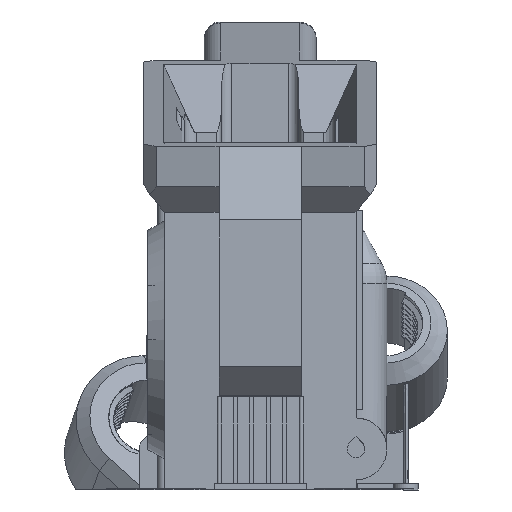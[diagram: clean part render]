
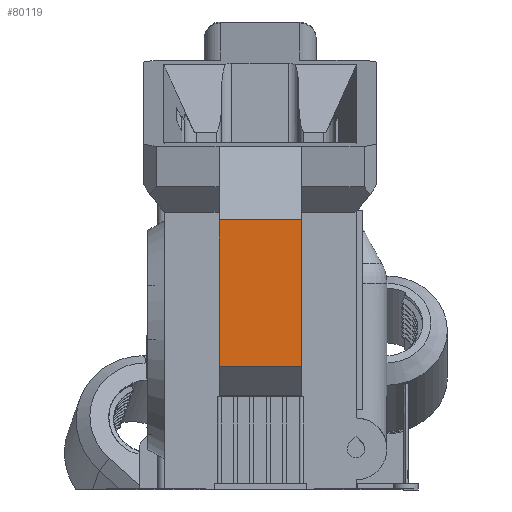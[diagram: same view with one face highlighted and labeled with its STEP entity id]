
A CAD part, left-side view. The second image highlights one B-rep face of the part: STEP entity #80119.
In plain terms, the highlighted planar face has unit normal (-1, 0, 0).
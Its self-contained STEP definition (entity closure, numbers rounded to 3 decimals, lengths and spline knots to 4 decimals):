
#517 = DIRECTION ( 'NONE',  ( 0., 0., 1. ) ) ;
#813 = EDGE_CURVE ( 'NONE', #81451, #173788, #107003, .T. ) ;
#8181 = VERTEX_POINT ( 'NONE', #47646 ) ;
#12141 = LINE ( 'NONE', #158535, #50473 ) ;
#12350 = DIRECTION ( 'NONE',  ( 0., 1., 0. ) ) ;
#18796 = EDGE_CURVE ( 'NONE', #173788, #8181, #12141, .T. ) ;
#22672 = CARTESIAN_POINT ( 'NONE',  ( -4.237, 1.1526, 2.4712 ) ) ;
#30576 = VERTEX_POINT ( 'NONE', #22672 ) ;
#31187 = VECTOR ( 'NONE', #92344, 39.3701 ) ;
#45227 = DIRECTION ( 'NONE',  ( -1., 0., 0. ) ) ;
#45407 = DIRECTION ( 'NONE',  ( 0., -1., 0. ) ) ;
#47646 = CARTESIAN_POINT ( 'NONE',  ( -4.237, 1.1526, 1.5782 ) ) ;
#47701 = CARTESIAN_POINT ( 'NONE',  ( -4.237, 1.1526, 1.5282 ) ) ;
#50473 = VECTOR ( 'NONE', #12350, 39.3701 ) ;
#51440 = CARTESIAN_POINT ( 'NONE',  ( -4.237, 0.6526, 1.5282 ) ) ;
#55194 = DIRECTION ( 'NONE',  ( 0., 0., -1. ) ) ;
#65679 = ORIENTED_EDGE ( 'NONE', *, *, #96995, .F. ) ;
#72227 = CARTESIAN_POINT ( 'NONE',  ( -4.237, 0.6526, 1.5782 ) ) ;
#80004 = VECTOR ( 'NONE', #55194, 39.3701 ) ;
#80119 = ADVANCED_FACE ( 'NONE', ( #184834 ), #131538, .T. ) ;
#81451 = VERTEX_POINT ( 'NONE', #146754 ) ;
#81904 = EDGE_LOOP ( 'NONE', ( #82337, #177744, #118762, #65679 ) ) ;
#82337 = ORIENTED_EDGE ( 'NONE', *, *, #18796, .F. ) ;
#92344 = DIRECTION ( 'NONE',  ( 0., 0., 1. ) ) ;
#96995 = EDGE_CURVE ( 'NONE', #8181, #30576, #184603, .T. ) ;
#107003 = LINE ( 'NONE', #51440, #80004 ) ;
#110475 = EDGE_CURVE ( 'NONE', #30576, #81451, #169175, .T. ) ;
#118762 = ORIENTED_EDGE ( 'NONE', *, *, #110475, .F. ) ;
#130163 = AXIS2_PLACEMENT_3D ( 'NONE', #159930, #45227, #517 ) ;
#131538 = PLANE ( 'NONE',  #130163 ) ;
#131732 = CARTESIAN_POINT ( 'NONE',  ( -4.237, 2.4558, 2.4712 ) ) ;
#137694 = VECTOR ( 'NONE', #45407, 39.3701 ) ;
#146754 = CARTESIAN_POINT ( 'NONE',  ( -4.237, 0.6526, 2.4712 ) ) ;
#158535 = CARTESIAN_POINT ( 'NONE',  ( -4.237, 2.4558, 1.5782 ) ) ;
#159930 = CARTESIAN_POINT ( 'NONE',  ( -4.237, 2.4558, 1.5282 ) ) ;
#169175 = LINE ( 'NONE', #131732, #137694 ) ;
#173788 = VERTEX_POINT ( 'NONE', #72227 ) ;
#177744 = ORIENTED_EDGE ( 'NONE', *, *, #813, .F. ) ;
#184603 = LINE ( 'NONE', #47701, #31187 ) ;
#184834 = FACE_OUTER_BOUND ( 'NONE', #81904, .T. ) ;
